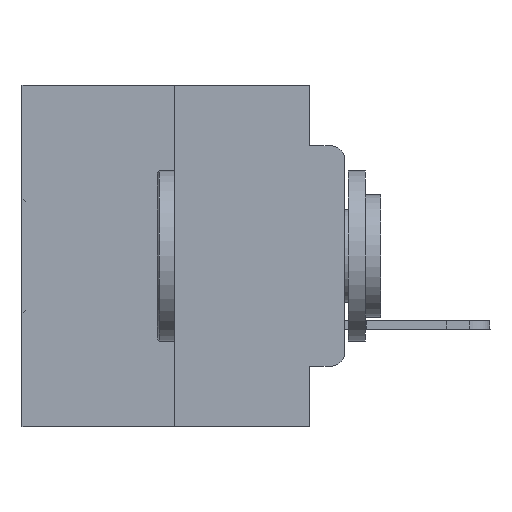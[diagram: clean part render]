
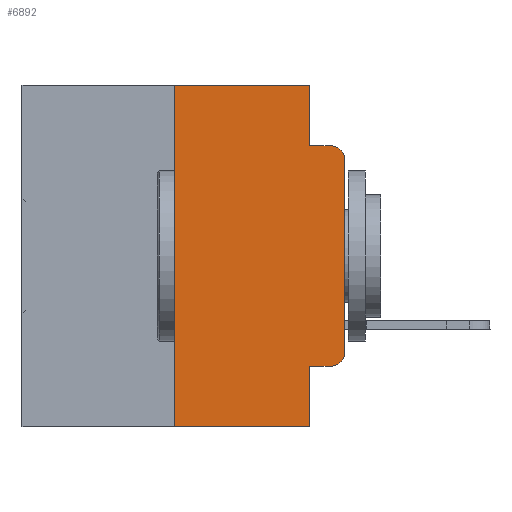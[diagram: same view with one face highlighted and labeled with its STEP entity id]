
A CAD part, left-side view. The second image highlights one B-rep face of the part: STEP entity #6892.
In plain terms, the highlighted planar face has unit normal (-1, 0, 0).
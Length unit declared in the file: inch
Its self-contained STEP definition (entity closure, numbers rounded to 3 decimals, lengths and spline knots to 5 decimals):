
#117 = VECTOR ( 'NONE', #7748, 39.37008 ) ;
#425 = DIRECTION ( 'NONE',  ( 0., 0., 1. ) ) ;
#636 = CARTESIAN_POINT ( 'NONE',  ( 0., 0., -0.1085 ) ) ;
#1093 = ORIENTED_EDGE ( 'NONE', *, *, #20535, .F. ) ;
#2026 = AXIS2_PLACEMENT_3D ( 'NONE', #27441, #15146, #19802 ) ;
#2332 = LINE ( 'NONE', #19239, #6641 ) ;
#2377 = EDGE_CURVE ( 'NONE', #32399, #15730, #18205, .T. ) ;
#2585 = VERTEX_POINT ( 'NONE', #19019 ) ;
#2642 = LINE ( 'NONE', #23492, #117 ) ;
#3671 = VECTOR ( 'NONE', #8744, 39.37008 ) ;
#3925 = CARTESIAN_POINT ( 'NONE',  ( 0., 0.051, 0. ) ) ;
#4326 = CARTESIAN_POINT ( 'NONE',  ( 0., 0., -0.3915 ) ) ;
#4777 = EDGE_CURVE ( 'NONE', #27231, #15872, #8110, .T. ) ;
#5478 = DIRECTION ( 'NONE',  ( 0., 0., 1. ) ) ;
#5581 = CARTESIAN_POINT ( 'NONE',  ( 0., 0.051, -0.5 ) ) ;
#5794 = CARTESIAN_POINT ( 'NONE',  ( 0., 0., 0. ) ) ;
#5983 = AXIS2_PLACEMENT_3D ( 'NONE', #10705, #8202, #19316 ) ;
#6641 = VECTOR ( 'NONE', #11776, 39.37008 ) ;
#6892 = ADVANCED_FACE ( 'NONE', ( #23302 ), #30932, .F. ) ;
#7197 = CARTESIAN_POINT ( 'NONE',  ( 0., 0.02, -0.4115 ) ) ;
#7748 = DIRECTION ( 'NONE',  ( 0., 0., -1. ) ) ;
#8110 = LINE ( 'NONE', #5794, #10199 ) ;
#8202 = DIRECTION ( 'NONE',  ( 1., 0., 0. ) ) ;
#8688 = VECTOR ( 'NONE', #425, 39.37008 ) ;
#8744 = DIRECTION ( 'NONE',  ( 0., 0., -1. ) ) ;
#8866 = CARTESIAN_POINT ( 'NONE',  ( 0., 0.25, -0.5 ) ) ;
#9050 = LINE ( 'NONE', #19167, #30290 ) ;
#9096 = EDGE_CURVE ( 'NONE', #10840, #15730, #9050, .T. ) ;
#10199 = VECTOR ( 'NONE', #5478, 39.37008 ) ;
#10309 = EDGE_CURVE ( 'NONE', #17292, #11426, #2642, .T. ) ;
#10705 = CARTESIAN_POINT ( 'NONE',  ( 0., 0.473, 0. ) ) ;
#10840 = VERTEX_POINT ( 'NONE', #8866 ) ;
#11134 = ORIENTED_EDGE ( 'NONE', *, *, #10309, .F. ) ;
#11380 = ORIENTED_EDGE ( 'NONE', *, *, #27272, .T. ) ;
#11413 = VERTEX_POINT ( 'NONE', #29876 ) ;
#11426 = VERTEX_POINT ( 'NONE', #12134 ) ;
#11471 = LINE ( 'NONE', #21581, #32115 ) ;
#11776 = DIRECTION ( 'NONE',  ( 0., -1., 0. ) ) ;
#12134 = CARTESIAN_POINT ( 'NONE',  ( 0., 0.051, -0.0885 ) ) ;
#12843 = LINE ( 'NONE', #32584, #25019 ) ;
#13066 = VERTEX_POINT ( 'NONE', #7197 ) ;
#13724 = CARTESIAN_POINT ( 'NONE',  ( 0., 0.051, 0. ) ) ;
#13765 = EDGE_CURVE ( 'NONE', #11426, #11413, #2332, .T. ) ;
#15146 = DIRECTION ( 'NONE',  ( -1., 0., 0. ) ) ;
#15730 = VERTEX_POINT ( 'NONE', #5581 ) ;
#15872 = VERTEX_POINT ( 'NONE', #636 ) ;
#16270 = ORIENTED_EDGE ( 'NONE', *, *, #13765, .F. ) ;
#17292 = VERTEX_POINT ( 'NONE', #3925 ) ;
#17346 = CARTESIAN_POINT ( 'NONE',  ( 0., 0.051, -0.4115 ) ) ;
#18205 = LINE ( 'NONE', #13724, #3671 ) ;
#18835 = ORIENTED_EDGE ( 'NONE', *, *, #28063, .T. ) ;
#18889 = CIRCLE ( 'NONE', #19958, 0.02 ) ;
#19019 = CARTESIAN_POINT ( 'NONE',  ( 0., 0.25, 0. ) ) ;
#19167 = CARTESIAN_POINT ( 'NONE',  ( 0., 0.473, -0.5 ) ) ;
#19239 = CARTESIAN_POINT ( 'NONE',  ( 0., 0.051, -0.0885 ) ) ;
#19316 = DIRECTION ( 'NONE',  ( 0., 0., -1. ) ) ;
#19802 = DIRECTION ( 'NONE',  ( 0., 0., -1. ) ) ;
#19958 = AXIS2_PLACEMENT_3D ( 'NONE', #28473, #31263, #21319 ) ;
#19998 = CIRCLE ( 'NONE', #2026, 0.02 ) ;
#20535 = EDGE_CURVE ( 'NONE', #2585, #17292, #12843, .T. ) ;
#21180 = ORIENTED_EDGE ( 'NONE', *, *, #4777, .T. ) ;
#21319 = DIRECTION ( 'NONE',  ( 0., 0., -1. ) ) ;
#21581 = CARTESIAN_POINT ( 'NONE',  ( 0., 0.051, -0.4115 ) ) ;
#23102 = CARTESIAN_POINT ( 'NONE',  ( 0., 0.25, 0. ) ) ;
#23239 = EDGE_CURVE ( 'NONE', #10840, #2585, #30396, .T. ) ;
#23302 = FACE_OUTER_BOUND ( 'NONE', #28041, .T. ) ;
#23492 = CARTESIAN_POINT ( 'NONE',  ( 0., 0.051, 0. ) ) ;
#25019 = VECTOR ( 'NONE', #27783, 39.37008 ) ;
#25347 = ORIENTED_EDGE ( 'NONE', *, *, #2377, .F. ) ;
#26260 = EDGE_CURVE ( 'NONE', #13066, #27231, #18889, .T. ) ;
#26974 = ORIENTED_EDGE ( 'NONE', *, *, #26260, .T. ) ;
#27231 = VERTEX_POINT ( 'NONE', #4326 ) ;
#27272 = EDGE_CURVE ( 'NONE', #32399, #13066, #11471, .T. ) ;
#27441 = CARTESIAN_POINT ( 'NONE',  ( 0., 0.02, -0.1085 ) ) ;
#27783 = DIRECTION ( 'NONE',  ( 0., -1., 0. ) ) ;
#28041 = EDGE_LOOP ( 'NONE', ( #21180, #18835, #16270, #11134, #1093, #31101, #28830, #25347, #11380, #26974 ) ) ;
#28063 = EDGE_CURVE ( 'NONE', #15872, #11413, #19998, .T. ) ;
#28473 = CARTESIAN_POINT ( 'NONE',  ( 0., 0.02, -0.3915 ) ) ;
#28830 = ORIENTED_EDGE ( 'NONE', *, *, #9096, .T. ) ;
#29693 = DIRECTION ( 'NONE',  ( 0., -1., 0. ) ) ;
#29876 = CARTESIAN_POINT ( 'NONE',  ( 0., 0.02, -0.0885 ) ) ;
#30290 = VECTOR ( 'NONE', #31121, 39.37008 ) ;
#30396 = LINE ( 'NONE', #23102, #8688 ) ;
#30932 = PLANE ( 'NONE',  #5983 ) ;
#31101 = ORIENTED_EDGE ( 'NONE', *, *, #23239, .F. ) ;
#31121 = DIRECTION ( 'NONE',  ( 0., -1., 0. ) ) ;
#31263 = DIRECTION ( 'NONE',  ( -1., 0., 0. ) ) ;
#32115 = VECTOR ( 'NONE', #29693, 39.37008 ) ;
#32399 = VERTEX_POINT ( 'NONE', #17346 ) ;
#32584 = CARTESIAN_POINT ( 'NONE',  ( 0., 0.473, 0. ) ) ;
